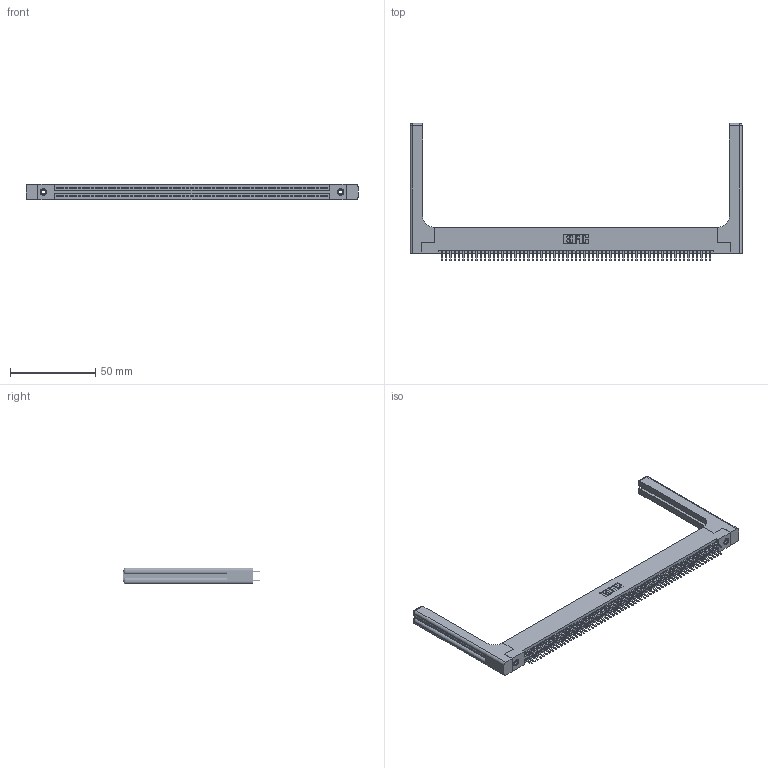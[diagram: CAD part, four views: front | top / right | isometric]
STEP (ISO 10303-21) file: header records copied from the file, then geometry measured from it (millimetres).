
FILE_DESCRIPTION (( 'STEP AP203' ), '1' );
FILE_NAME ('395-126-520-258.STEP', '2019-10-28T13:43:58', ( '' ), ( '' ), 'SwSTEP 2.0', 'SolidWorks 2016', '' );
FILE_SCHEMA (( 'CONFIG_CONTROL_DESIGN' ));
Length unit declared in the file: inch
Products named in the file (5): 345-292-001_345-293-120; 345-250-001_345-250-001-102; 345-220-058_345-220-058; 395-126-520-258; 345 Part_Flush Mounting Lugs - 0.156 Dia-TH
Assembly tree (131 placements, depth 2):
  395-126-520-258
    345 Part_Flush Mounting Lugs - 0.156 Dia-TH
    345-292-001_345-293-120  x126
    345-250-001_345-250-001-102  x2
    345-220-058_345-220-058  x2
Bounding box: 195.05 x 80.64 x 9.4 mm (x, y, z)
Volume: 27561.7 mm3; surface area: 33560.9 mm2
Topology: 131 solids, 131 shells, 7186 faces, 20789 edges, 13502 vertices
Faces by surface type: plane 4638, cylinder 2488, bspline 36, cone 12, sphere 8, torus 4
Entity records: 51900 total; most frequent: CARTESIAN_POINT 9685, ORIENTED_EDGE 8404, DIRECTION 7434, EDGE_CURVE 4202, VECTOR 3722, LINE 3722, VERTEX_POINT 2790, AXIS2_PLACEMENT_3D 1856
